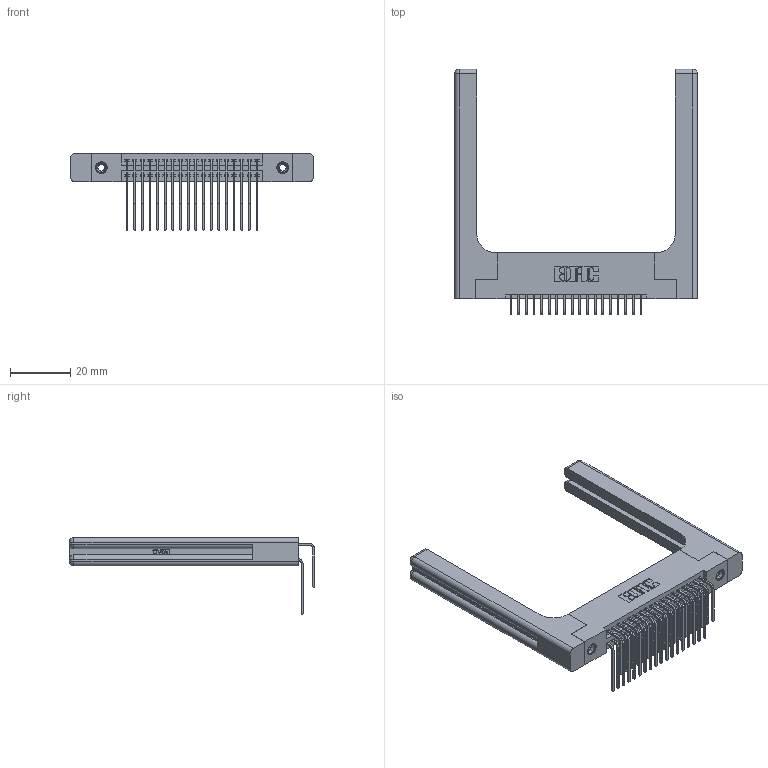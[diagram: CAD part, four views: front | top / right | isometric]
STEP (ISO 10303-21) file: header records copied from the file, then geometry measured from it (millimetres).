
FILE_DESCRIPTION (( 'STEP AP203' ), '1' );
FILE_NAME ('395-036-559-258.STEP', '2019-10-18T03:03:32', ( '' ), ( '' ), 'SwSTEP 2.0', 'SolidWorks 2016', '' );
FILE_SCHEMA (( 'CONFIG_CONTROL_DESIGN' ));
Length unit declared in the file: inch
Products named in the file (6): 345-292-001_559 Tail - 2; 345-250-001_345-250-001-102; 345-220-058_345-220-058; 395-036-559-258; 345 Part_Flush Mounting Lugs - 0.156 Dia-TH; 345-292-001_558 559 Tail - 1
Assembly tree (41 placements, depth 2):
  395-036-559-258
    345 Part_Flush Mounting Lugs - 0.156 Dia-TH
    345-292-001_558 559 Tail - 1  x18
    345-292-001_559 Tail - 2  x18
    345-250-001_345-250-001-102  x2
    345-220-058_345-220-058  x2
Bounding box: 80.75 x 81.52 x 25.53 mm (x, y, z)
Volume: 16303.8 mm3; surface area: 17142.7 mm2
Topology: 41 solids, 41 shells, 2254 faces, 6587 edges, 4322 vertices
Faces by surface type: plane 1488, cylinder 706, bspline 36, cone 12, sphere 8, torus 4
Entity records: 24188 total; most frequent: CARTESIAN_POINT 5116, ORIENTED_EDGE 3796, DIRECTION 3446, EDGE_CURVE 1898, LINE 1562, VECTOR 1562, VERTEX_POINT 1254, AXIS2_PLACEMENT_3D 942
